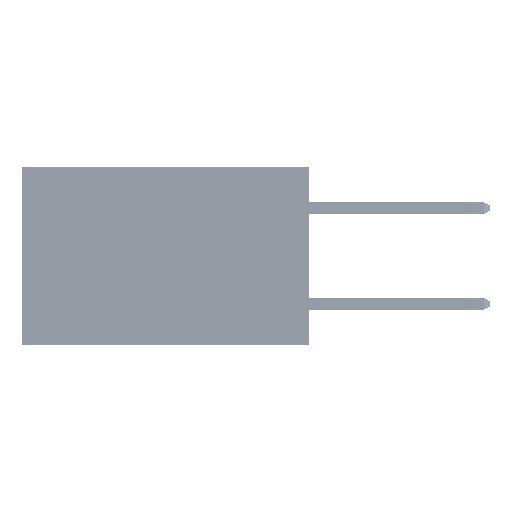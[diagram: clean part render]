
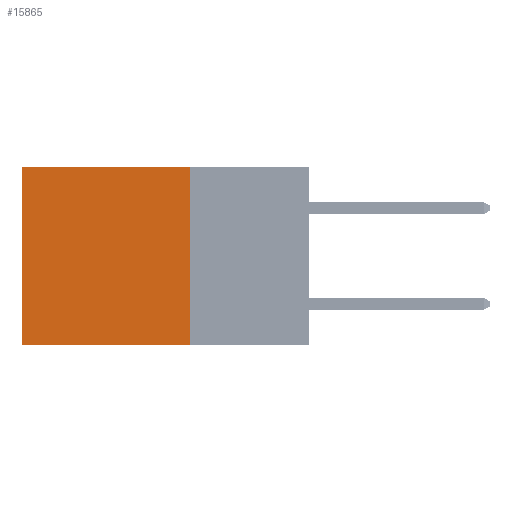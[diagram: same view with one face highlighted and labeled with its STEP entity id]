
A CAD part, left-side view. The second image highlights one B-rep face of the part: STEP entity #15865.
In plain terms, the highlighted planar face has unit normal (-1, 0, 0).
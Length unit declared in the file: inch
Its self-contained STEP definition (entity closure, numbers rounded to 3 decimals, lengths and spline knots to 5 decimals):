
#2013 = AXIS2_PLACEMENT_3D ( 'NONE', #11603, #27373, #6721 ) ;
#2620 = DIRECTION ( 'NONE',  ( 0., 1., 0. ) ) ;
#2871 = PLANE ( 'NONE',  #2013 ) ;
#3613 = DIRECTION ( 'NONE',  ( 0., 1., 0. ) ) ;
#4589 = CARTESIAN_POINT ( 'NONE',  ( 0.2875, 0.6, -0.37 ) ) ;
#5922 = VERTEX_POINT ( 'NONE', #30411 ) ;
#6721 = DIRECTION ( 'NONE',  ( 0., 0., -1. ) ) ;
#7374 = VERTEX_POINT ( 'NONE', #23042 ) ;
#8360 = CARTESIAN_POINT ( 'NONE',  ( 0.2875, 0.6, 0. ) ) ;
#8553 = VERTEX_POINT ( 'NONE', #49384 ) ;
#9948 = EDGE_LOOP ( 'NONE', ( #34121, #10246, #37998, #32156 ) ) ;
#10246 = ORIENTED_EDGE ( 'NONE', *, *, #48887, .F. ) ;
#11603 = CARTESIAN_POINT ( 'NONE',  ( 0.2875, 0.25, 0. ) ) ;
#12140 = LINE ( 'NONE', #31493, #38456 ) ;
#15865 = ADVANCED_FACE ( 'NONE', ( #42095 ), #2871, .F. ) ;
#16399 = LINE ( 'NONE', #8360, #35167 ) ;
#21605 = VERTEX_POINT ( 'NONE', #4589 ) ;
#21745 = LINE ( 'NONE', #22255, #38293 ) ;
#22255 = CARTESIAN_POINT ( 'NONE',  ( 0.2875, 0.25, 0. ) ) ;
#22715 = EDGE_CURVE ( 'NONE', #7374, #8553, #21745, .T. ) ;
#23042 = CARTESIAN_POINT ( 'NONE',  ( 0.2875, 0.25, 0. ) ) ;
#25177 = EDGE_CURVE ( 'NONE', #8553, #21605, #16399, .T. ) ;
#27373 = DIRECTION ( 'NONE',  ( 1., 0., 0. ) ) ;
#30411 = CARTESIAN_POINT ( 'NONE',  ( 0.2875, 0.25, -0.37 ) ) ;
#31493 = CARTESIAN_POINT ( 'NONE',  ( 0.2875, 0.25, -0.37 ) ) ;
#32141 = DIRECTION ( 'NONE',  ( 0., 0., -1. ) ) ;
#32156 = ORIENTED_EDGE ( 'NONE', *, *, #22715, .T. ) ;
#34121 = ORIENTED_EDGE ( 'NONE', *, *, #25177, .T. ) ;
#35167 = VECTOR ( 'NONE', #32141, 39.37008 ) ;
#35889 = DIRECTION ( 'NONE',  ( 0., 0., -1. ) ) ;
#36012 = EDGE_CURVE ( 'NONE', #7374, #5922, #47756, .T. ) ;
#36149 = CARTESIAN_POINT ( 'NONE',  ( 0.2875, 0.25, 0. ) ) ;
#37998 = ORIENTED_EDGE ( 'NONE', *, *, #36012, .F. ) ;
#38293 = VECTOR ( 'NONE', #2620, 39.37008 ) ;
#38456 = VECTOR ( 'NONE', #3613, 39.37008 ) ;
#42095 = FACE_OUTER_BOUND ( 'NONE', #9948, .T. ) ;
#46400 = VECTOR ( 'NONE', #35889, 39.37008 ) ;
#47756 = LINE ( 'NONE', #36149, #46400 ) ;
#48887 = EDGE_CURVE ( 'NONE', #5922, #21605, #12140, .T. ) ;
#49384 = CARTESIAN_POINT ( 'NONE',  ( 0.2875, 0.6, 0. ) ) ;
